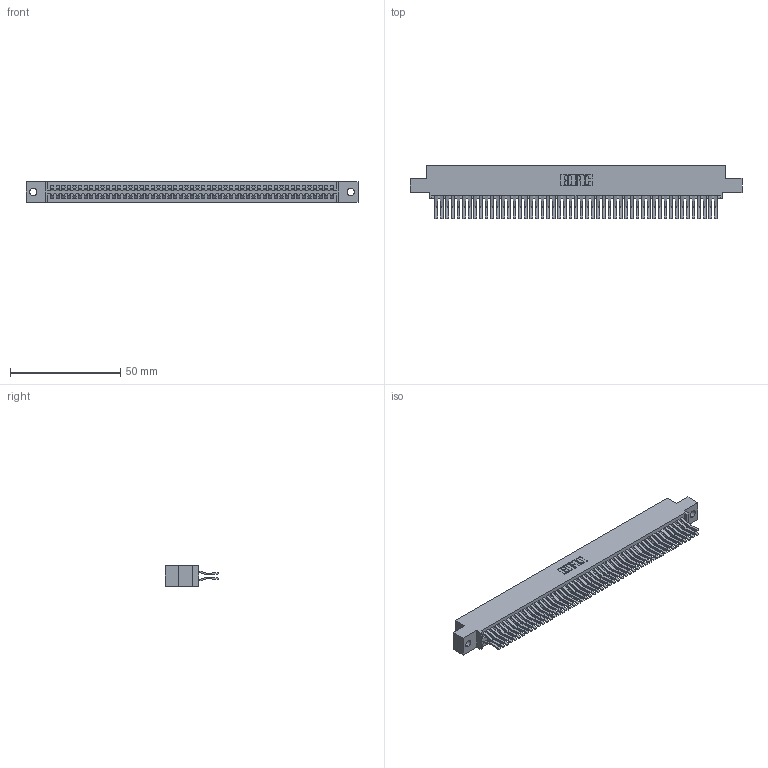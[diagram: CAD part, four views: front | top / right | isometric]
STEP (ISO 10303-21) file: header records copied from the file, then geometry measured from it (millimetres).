
FILE_DESCRIPTION (( 'STEP AP203' ), '1' );
FILE_NAME ('345-102-560-502.STEP', '2018-10-05T21:51:49', ( '' ), ( '' ), 'SwSTEP 2.0', 'SolidWorks 2016', '' );
FILE_SCHEMA (( 'CONFIG_CONTROL_DESIGN' ));
Length unit declared in the file: inch
Products named in the file (3): 345-102-560-502; 345-292-001_560 Tail; 345 Part_0.110 Offset - 0.128 Dia
Assembly tree (103 placements, depth 2):
  345-102-560-502
    345 Part_0.110 Offset - 0.128 Dia
    345-292-001_560 Tail  x102
Bounding box: 150.75 x 24.45 x 9.4 mm (x, y, z)
Volume: 15286 mm3; surface area: 24309.2 mm2
Topology: 103 solids, 103 shells, 5434 faces, 16163 edges, 10638 vertices
Faces by surface type: plane 3450, cylinder 1984
Entity records: 39027 total; most frequent: CARTESIAN_POINT 6536, ORIENTED_EDGE 6470, DIRECTION 5755, EDGE_CURVE 3235, LINE 2895, VECTOR 2895, VERTEX_POINT 2154, AXIS2_PLACEMENT_3D 1430
